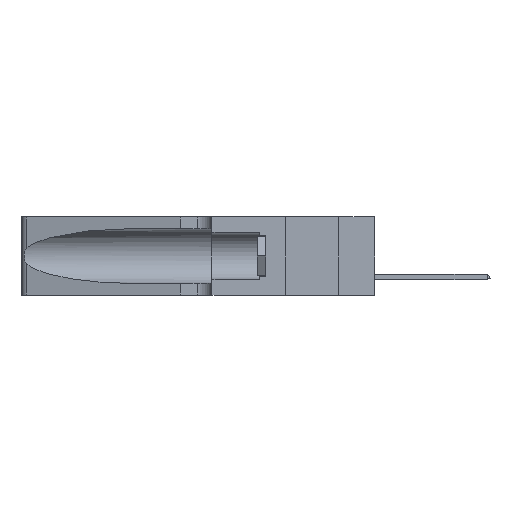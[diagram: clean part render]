
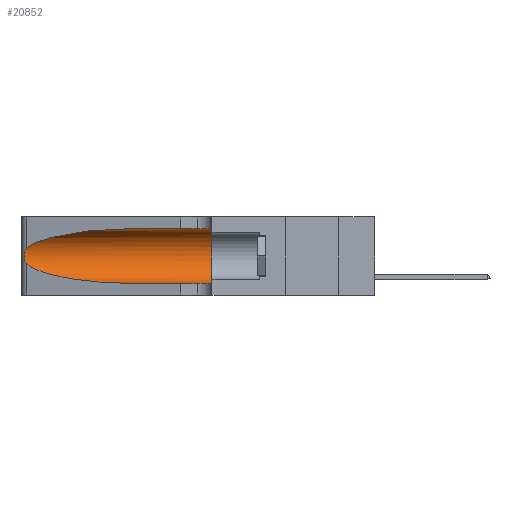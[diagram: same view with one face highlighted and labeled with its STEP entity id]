
A CAD part, left-side view. The second image highlights one B-rep face of the part: STEP entity #20852.
In plain terms, the highlighted cylindrical face has radius 3.308 mm (diameter 6.617 mm), a partial arc.
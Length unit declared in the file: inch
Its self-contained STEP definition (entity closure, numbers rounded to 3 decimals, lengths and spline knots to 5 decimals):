
#556 = CARTESIAN_POINT ( 'NONE',  ( 0.1305, 0.35, 0.185 ) ) ;
#606 = EDGE_LOOP ( 'NONE', ( #42164, #37782, #12934, #20118, #31193, #27040 ) ) ;
#1034 = CARTESIAN_POINT ( 'NONE',  ( 0.1305, 0.35, 0.31525 ) ) ;
#1600 = EDGE_CURVE ( 'NONE', #44535, #47475, #7572, .T. ) ;
#3318 = LINE ( 'NONE', #48153, #15267 ) ;
#3620 = VERTEX_POINT ( 'NONE', #37513 ) ;
#5983 = DIRECTION ( 'NONE',  ( 0., -1., 0. ) ) ;
#6103 = VERTEX_POINT ( 'NONE', #14154 ) ;
#6111 = EDGE_CURVE ( 'NONE', #6103, #24590, #35738, .T. ) ;
#6414 = FACE_OUTER_BOUND ( 'NONE', #606, .T. ) ;
#7572 =( BOUNDED_CURVE ( )  B_SPLINE_CURVE ( 3, ( #44751, #10779, #21985, #22797 ),
 .UNSPECIFIED., .F., .F. ) 
 B_SPLINE_CURVE_WITH_KNOTS ( ( 4, 4 ),
 ( 3.44316, 4.71239 ),
 .UNSPECIFIED. ) 
 CURVE ( )  GEOMETRIC_REPRESENTATION_ITEM ( )  RATIONAL_B_SPLINE_CURVE ( ( 1., 0.87, 0.87, 1. ) ) 
 REPRESENTATION_ITEM ( '' )  );
#7816 = VERTEX_POINT ( 'NONE', #13703 ) ;
#7934 = DIRECTION ( 'NONE',  ( 0., 0., 1. ) ) ;
#8071 = CARTESIAN_POINT ( 'NONE',  ( 0.25555, 1.22994, 0.2215 ) ) ;
#10779 = CARTESIAN_POINT ( 'NONE',  ( 0.2373, 1.15595, 0.08982 ) ) ;
#10854 = EDGE_CURVE ( 'NONE', #7816, #44535, #41796, .T. ) ;
#11501 = CARTESIAN_POINT ( 'NONE',  ( 0.26018, 1.23835, 0.19895 ) ) ;
#12934 = ORIENTED_EDGE ( 'NONE', *, *, #1600, .T. ) ;
#13155 = CARTESIAN_POINT ( 'NONE',  ( 0.2373, 1.15595, 0.28018 ) ) ;
#13703 = CARTESIAN_POINT ( 'NONE',  ( 0.25487, 1.22718, 0.22369 ) ) ;
#14154 = CARTESIAN_POINT ( 'NONE',  ( 0.1305, 0.72297, 0.31525 ) ) ;
#15267 = VECTOR ( 'NONE', #5983, 39.37008 ) ;
#15299 = CARTESIAN_POINT ( 'NONE',  ( 0.26075, 1.23896, 0.178 ) ) ;
#16882 = CARTESIAN_POINT ( 'NONE',  ( 0.1305, 0.72297, 0.05475 ) ) ;
#16967 = CARTESIAN_POINT ( 'NONE',  ( 0.25487, 1.22718, 0.22369 ) ) ;
#19176 = CARTESIAN_POINT ( 'NONE',  ( 0.25639, 1.23184, 0.21858 ) ) ;
#19380 = CIRCLE ( 'NONE', #47176, 0.13025 ) ;
#20118 = ORIENTED_EDGE ( 'NONE', *, *, #43113, .T. ) ;
#20852 = ADVANCED_FACE ( 'NONE', ( #6414 ), #38627, .F. ) ;
#21985 = CARTESIAN_POINT ( 'NONE',  ( 0.18966, 0.96281, 0.05475 ) ) ;
#22797 = CARTESIAN_POINT ( 'NONE',  ( 0.1305, 0.72297, 0.05475 ) ) ;
#23021 = CARTESIAN_POINT ( 'NONE',  ( 0.25856, 1.23593, 0.16098 ) ) ;
#24170 = EDGE_CURVE ( 'NONE', #6103, #7816, #32011, .T. ) ;
#24590 = VERTEX_POINT ( 'NONE', #1034 ) ;
#25567 = CARTESIAN_POINT ( 'NONE',  ( 0.1305, 1.61858, 0.185 ) ) ;
#25633 = CARTESIAN_POINT ( 'NONE',  ( 0.1305, 1.61858, 0.31525 ) ) ;
#26640 = CARTESIAN_POINT ( 'NONE',  ( 0.25854, 1.2359, 0.20912 ) ) ;
#27040 = ORIENTED_EDGE ( 'NONE', *, *, #6111, .F. ) ;
#27259 = DIRECTION ( 'NONE',  ( 0., 1., 0. ) ) ;
#30314 = CARTESIAN_POINT ( 'NONE',  ( 0.25487, 1.22718, 0.22369 ) ) ;
#30626 = CARTESIAN_POINT ( 'NONE',  ( 0.25555, 1.22993, 0.14849 ) ) ;
#30923 = CARTESIAN_POINT ( 'NONE',  ( 0.25789, 1.23486, 0.15765 ) ) ;
#31193 = ORIENTED_EDGE ( 'NONE', *, *, #34675, .F. ) ;
#32011 =( BOUNDED_CURVE ( )  B_SPLINE_CURVE ( 3, ( #42939, #35957, #13155, #16967 ),
 .UNSPECIFIED., .F., .F. ) 
 B_SPLINE_CURVE_WITH_KNOTS ( ( 4, 4 ),
 ( 1.5708, 2.84003 ),
 .UNSPECIFIED. ) 
 CURVE ( )  GEOMETRIC_REPRESENTATION_ITEM ( )  RATIONAL_B_SPLINE_CURVE ( ( 1., 0.87, 0.87, 1. ) ) 
 REPRESENTATION_ITEM ( '' )  );
#34444 = CARTESIAN_POINT ( 'NONE',  ( 0.25639, 1.23186, 0.15144 ) ) ;
#34675 = EDGE_CURVE ( 'NONE', #24590, #3620, #19380, .T. ) ;
#35738 = LINE ( 'NONE', #25633, #45317 ) ;
#35957 = CARTESIAN_POINT ( 'NONE',  ( 0.18966, 0.96281, 0.31525 ) ) ;
#37513 = CARTESIAN_POINT ( 'NONE',  ( 0.1305, 0.35, 0.05475 ) ) ;
#37782 = ORIENTED_EDGE ( 'NONE', *, *, #10854, .T. ) ;
#38472 = CARTESIAN_POINT ( 'NONE',  ( 0.26075, 1.23896, 0.19203 ) ) ;
#38627 = CYLINDRICAL_SURFACE ( 'NONE', #38800, 0.13025 ) ;
#38800 = AXIS2_PLACEMENT_3D ( 'NONE', #25567, #44206, #45519 ) ;
#40806 = DIRECTION ( 'NONE',  ( 0., -1., 0. ) ) ;
#41666 = CARTESIAN_POINT ( 'NONE',  ( 0.25487, 1.22718, 0.14631 ) ) ;
#41796 = B_SPLINE_CURVE_WITH_KNOTS ( 'NONE', 3,
 ( #30314, #8071, #19176, #41823, #26640, #11501, #38472, #15299, #45782, #23021, #30923, #34444, #30626, #46099 ),
 .UNSPECIFIED., .F., .F.,
 ( 4, 2, 2, 2, 2, 2, 4 ),
 ( 0., 0.00027, 0.00053, 0.00107, 0.0016, 0.00187, 0.00214 ),
 .UNSPECIFIED. ) ;
#41823 = CARTESIAN_POINT ( 'NONE',  ( 0.25787, 1.23484, 0.2124 ) ) ;
#42164 = ORIENTED_EDGE ( 'NONE', *, *, #24170, .T. ) ;
#42939 = CARTESIAN_POINT ( 'NONE',  ( 0.1305, 0.72297, 0.31525 ) ) ;
#43113 = EDGE_CURVE ( 'NONE', #47475, #3620, #3318, .T. ) ;
#44206 = DIRECTION ( 'NONE',  ( 0., -1., 0. ) ) ;
#44535 = VERTEX_POINT ( 'NONE', #41666 ) ;
#44751 = CARTESIAN_POINT ( 'NONE',  ( 0.25487, 1.22718, 0.14631 ) ) ;
#45317 = VECTOR ( 'NONE', #40806, 39.37008 ) ;
#45519 = DIRECTION ( 'NONE',  ( 0., 0., -1. ) ) ;
#45782 = CARTESIAN_POINT ( 'NONE',  ( 0.26017, 1.23833, 0.17102 ) ) ;
#46099 = CARTESIAN_POINT ( 'NONE',  ( 0.25487, 1.22718, 0.14631 ) ) ;
#47176 = AXIS2_PLACEMENT_3D ( 'NONE', #556, #27259, #7934 ) ;
#47475 = VERTEX_POINT ( 'NONE', #16882 ) ;
#48153 = CARTESIAN_POINT ( 'NONE',  ( 0.1305, 1.61858, 0.05475 ) ) ;
